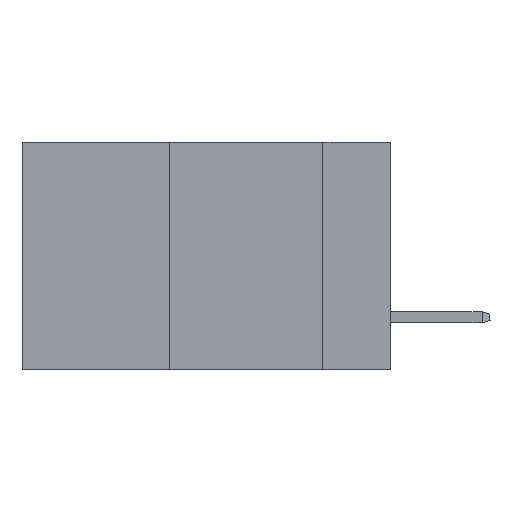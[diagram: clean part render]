
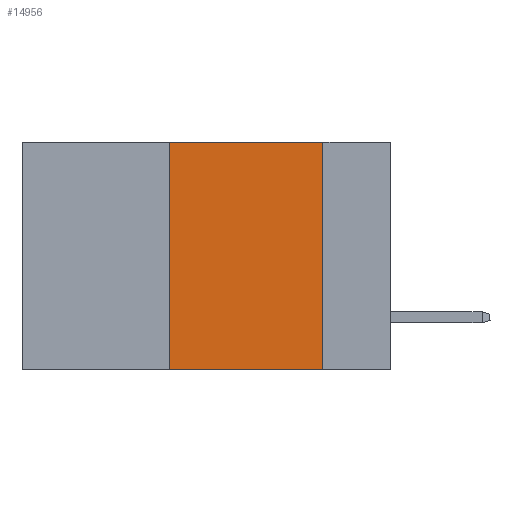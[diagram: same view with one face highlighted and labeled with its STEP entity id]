
A CAD part, left-side view. The second image highlights one B-rep face of the part: STEP entity #14956.
In plain terms, the highlighted planar face has unit normal (-1, 0, 0).
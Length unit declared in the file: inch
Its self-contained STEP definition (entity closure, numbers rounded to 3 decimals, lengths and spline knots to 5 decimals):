
#319 = CARTESIAN_POINT ( 'NONE',  ( 0., 0.6, 0. ) ) ;
#2877 = DIRECTION ( 'NONE',  ( 0., 0., -1. ) ) ;
#2987 = VECTOR ( 'NONE', #29842, 39.37008 ) ;
#3069 = EDGE_LOOP ( 'NONE', ( #36232, #27909, #6594, #31434 ) ) ;
#4338 = FACE_OUTER_BOUND ( 'NONE', #3069, .T. ) ;
#5554 = CARTESIAN_POINT ( 'NONE',  ( 0., 0.6, 0. ) ) ;
#6594 = ORIENTED_EDGE ( 'NONE', *, *, #9566, .F. ) ;
#7456 = VECTOR ( 'NONE', #16676, 39.37008 ) ;
#9414 = CARTESIAN_POINT ( 'NONE',  ( 0., 0.11, 0. ) ) ;
#9566 = EDGE_CURVE ( 'NONE', #25504, #26244, #37554, .T. ) ;
#12297 = LINE ( 'NONE', #13610, #7456 ) ;
#12329 = CARTESIAN_POINT ( 'NONE',  ( 0., 0.6, -0.37 ) ) ;
#13610 = CARTESIAN_POINT ( 'NONE',  ( 0., 0.11, 0. ) ) ;
#14956 = ADVANCED_FACE ( 'NONE', ( #4338 ), #38898, .F. ) ;
#16676 = DIRECTION ( 'NONE',  ( 0., 0., -1. ) ) ;
#20083 = VECTOR ( 'NONE', #37406, 39.37008 ) ;
#21211 = EDGE_CURVE ( 'NONE', #26244, #26698, #36429, .T. ) ;
#21679 = DIRECTION ( 'NONE',  ( 0., -1., 0. ) ) ;
#22147 = LINE ( 'NONE', #12329, #31271 ) ;
#23813 = CARTESIAN_POINT ( 'NONE',  ( 0., 0.36, 0. ) ) ;
#25504 = VERTEX_POINT ( 'NONE', #36825 ) ;
#26244 = VERTEX_POINT ( 'NONE', #38294 ) ;
#26698 = VERTEX_POINT ( 'NONE', #9414 ) ;
#27261 = AXIS2_PLACEMENT_3D ( 'NONE', #5554, #33223, #2877 ) ;
#27909 = ORIENTED_EDGE ( 'NONE', *, *, #21211, .F. ) ;
#29842 = DIRECTION ( 'NONE',  ( 0., 0., 1. ) ) ;
#31271 = VECTOR ( 'NONE', #21679, 39.37008 ) ;
#31434 = ORIENTED_EDGE ( 'NONE', *, *, #34187, .T. ) ;
#31634 = EDGE_CURVE ( 'NONE', #26698, #34170, #12297, .T. ) ;
#33223 = DIRECTION ( 'NONE',  ( 1., 0., 0. ) ) ;
#33367 = CARTESIAN_POINT ( 'NONE',  ( 0., 0.11, -0.37 ) ) ;
#34170 = VERTEX_POINT ( 'NONE', #33367 ) ;
#34187 = EDGE_CURVE ( 'NONE', #25504, #34170, #22147, .T. ) ;
#36232 = ORIENTED_EDGE ( 'NONE', *, *, #31634, .F. ) ;
#36429 = LINE ( 'NONE', #319, #20083 ) ;
#36825 = CARTESIAN_POINT ( 'NONE',  ( 0., 0.36, -0.37 ) ) ;
#37406 = DIRECTION ( 'NONE',  ( 0., -1., 0. ) ) ;
#37554 = LINE ( 'NONE', #23813, #2987 ) ;
#38294 = CARTESIAN_POINT ( 'NONE',  ( 0., 0.36, 0. ) ) ;
#38898 = PLANE ( 'NONE',  #27261 ) ;
